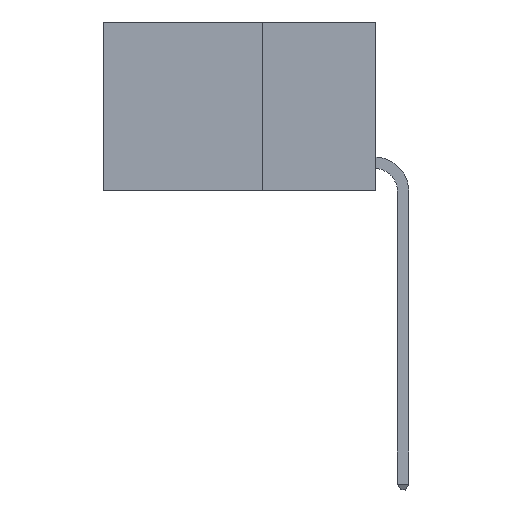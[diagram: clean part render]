
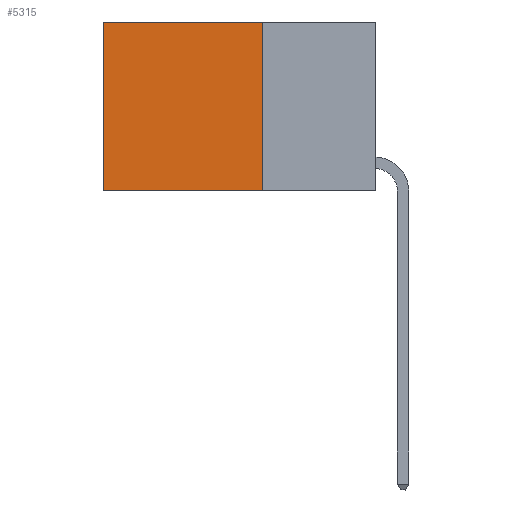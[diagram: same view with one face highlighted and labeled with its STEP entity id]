
A CAD part, left-side view. The second image highlights one B-rep face of the part: STEP entity #5315.
In plain terms, the highlighted planar face has unit normal (-1, 0, 0).
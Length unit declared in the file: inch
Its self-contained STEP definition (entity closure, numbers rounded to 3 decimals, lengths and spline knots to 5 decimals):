
#1024 = CARTESIAN_POINT ( 'NONE',  ( 0.2625, 0.25, 0. ) ) ;
#1442 = LINE ( 'NONE', #2452, #17322 ) ;
#2452 = CARTESIAN_POINT ( 'NONE',  ( 0.2625, 0.25, 0. ) ) ;
#2560 = VERTEX_POINT ( 'NONE', #16971 ) ;
#3117 = DIRECTION ( 'NONE',  ( 0., 0., -1. ) ) ;
#4074 = ORIENTED_EDGE ( 'NONE', *, *, #22422, .F. ) ;
#4805 = EDGE_LOOP ( 'NONE', ( #22002, #4074, #9711, #13241 ) ) ;
#5315 = ADVANCED_FACE ( 'NONE', ( #12569 ), #20813, .F. ) ;
#6540 = DIRECTION ( 'NONE',  ( 0., 1., 0. ) ) ;
#6597 = CARTESIAN_POINT ( 'NONE',  ( 0.2625, 0.6, 0. ) ) ;
#6893 = LINE ( 'NONE', #15743, #10888 ) ;
#7516 = DIRECTION ( 'NONE',  ( 0., 0., -1. ) ) ;
#9403 = LINE ( 'NONE', #6597, #19262 ) ;
#9711 = ORIENTED_EDGE ( 'NONE', *, *, #19421, .F. ) ;
#9889 = VERTEX_POINT ( 'NONE', #23854 ) ;
#10888 = VECTOR ( 'NONE', #21665, 39.37008 ) ;
#12569 = FACE_OUTER_BOUND ( 'NONE', #4805, .T. ) ;
#13241 = ORIENTED_EDGE ( 'NONE', *, *, #17291, .T. ) ;
#13321 = CARTESIAN_POINT ( 'NONE',  ( 0.2625, 0.25, 0. ) ) ;
#14086 = CARTESIAN_POINT ( 'NONE',  ( 0.2625, 0.25, -0.37 ) ) ;
#14962 = DIRECTION ( 'NONE',  ( 1., 0., 0. ) ) ;
#15455 = VERTEX_POINT ( 'NONE', #20354 ) ;
#15743 = CARTESIAN_POINT ( 'NONE',  ( 0.2625, 0.25, -0.37 ) ) ;
#16658 = VERTEX_POINT ( 'NONE', #14086 ) ;
#16971 = CARTESIAN_POINT ( 'NONE',  ( 0.2625, 0.6, 0. ) ) ;
#17195 = VECTOR ( 'NONE', #7516, 39.37008 ) ;
#17291 = EDGE_CURVE ( 'NONE', #9889, #2560, #1442, .T. ) ;
#17322 = VECTOR ( 'NONE', #6540, 39.37008 ) ;
#19262 = VECTOR ( 'NONE', #24209, 39.37008 ) ;
#19421 = EDGE_CURVE ( 'NONE', #9889, #16658, #22974, .T. ) ;
#19516 = AXIS2_PLACEMENT_3D ( 'NONE', #1024, #14962, #3117 ) ;
#20354 = CARTESIAN_POINT ( 'NONE',  ( 0.2625, 0.6, -0.37 ) ) ;
#20813 = PLANE ( 'NONE',  #19516 ) ;
#21477 = EDGE_CURVE ( 'NONE', #2560, #15455, #9403, .T. ) ;
#21665 = DIRECTION ( 'NONE',  ( 0., 1., 0. ) ) ;
#22002 = ORIENTED_EDGE ( 'NONE', *, *, #21477, .T. ) ;
#22422 = EDGE_CURVE ( 'NONE', #16658, #15455, #6893, .T. ) ;
#22974 = LINE ( 'NONE', #13321, #17195 ) ;
#23854 = CARTESIAN_POINT ( 'NONE',  ( 0.2625, 0.25, 0. ) ) ;
#24209 = DIRECTION ( 'NONE',  ( 0., 0., -1. ) ) ;
